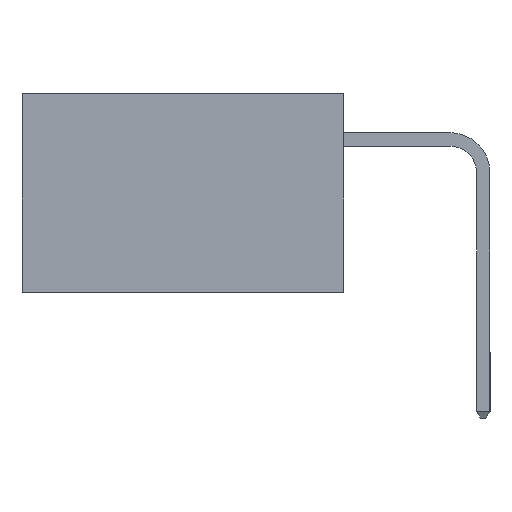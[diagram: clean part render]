
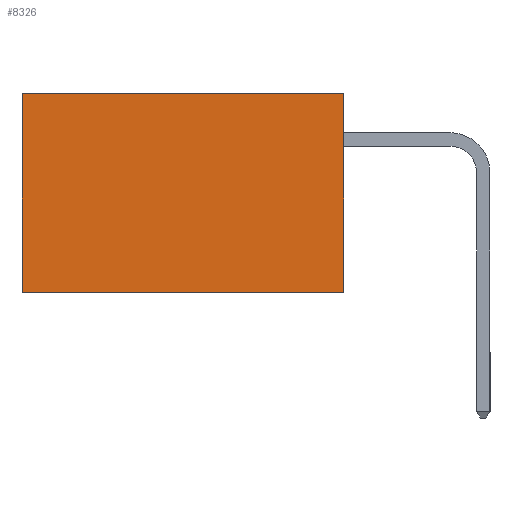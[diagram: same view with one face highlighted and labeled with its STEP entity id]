
A CAD part, left-side view. The second image highlights one B-rep face of the part: STEP entity #8326.
In plain terms, the highlighted planar face has unit normal (-1, 0, 0).
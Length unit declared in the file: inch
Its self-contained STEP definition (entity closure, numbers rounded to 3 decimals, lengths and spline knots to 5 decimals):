
#190 = ORIENTED_EDGE ( 'NONE', *, *, #11918, .T. ) ;
#529 = VECTOR ( 'NONE', #6124, 39.37008 ) ;
#577 = CARTESIAN_POINT ( 'NONE',  ( 0.2615, 0., -0.37 ) ) ;
#849 = LINE ( 'NONE', #4557, #6924 ) ;
#1777 = VERTEX_POINT ( 'NONE', #5618 ) ;
#2087 = DIRECTION ( 'NONE',  ( 0., 1., 0. ) ) ;
#2812 = VECTOR ( 'NONE', #5558, 39.37008 ) ;
#2943 = ORIENTED_EDGE ( 'NONE', *, *, #10441, .T. ) ;
#3021 = CARTESIAN_POINT ( 'NONE',  ( 0.2615, 0., -0.37 ) ) ;
#3603 = EDGE_CURVE ( 'NONE', #6421, #6858, #5610, .T. ) ;
#4172 = CARTESIAN_POINT ( 'NONE',  ( 0.2615, 0.6, -0.37 ) ) ;
#4557 = CARTESIAN_POINT ( 'NONE',  ( 0.2615, 0.6, -0.37 ) ) ;
#5007 = DIRECTION ( 'NONE',  ( 0., 0., -1. ) ) ;
#5544 = CARTESIAN_POINT ( 'NONE',  ( 0.2615, 0., -0.37 ) ) ;
#5558 = DIRECTION ( 'NONE',  ( 0., 0., -1. ) ) ;
#5610 = LINE ( 'NONE', #5544, #5855 ) ;
#5618 = CARTESIAN_POINT ( 'NONE',  ( 0.2615, 0.6, 0. ) ) ;
#5855 = VECTOR ( 'NONE', #2087, 39.37008 ) ;
#5917 = FACE_OUTER_BOUND ( 'NONE', #8085, .T. ) ;
#6124 = DIRECTION ( 'NONE',  ( 0., 1., 0. ) ) ;
#6421 = VERTEX_POINT ( 'NONE', #8128 ) ;
#6769 = ORIENTED_EDGE ( 'NONE', *, *, #8124, .F. ) ;
#6772 = PLANE ( 'NONE',  #7582 ) ;
#6858 = VERTEX_POINT ( 'NONE', #4172 ) ;
#6924 = VECTOR ( 'NONE', #8260, 39.37008 ) ;
#7440 = ORIENTED_EDGE ( 'NONE', *, *, #3603, .F. ) ;
#7582 = AXIS2_PLACEMENT_3D ( 'NONE', #3021, #8595, #5007 ) ;
#7611 = CARTESIAN_POINT ( 'NONE',  ( 0.2615, 0., 0. ) ) ;
#8015 = LINE ( 'NONE', #10806, #529 ) ;
#8085 = EDGE_LOOP ( 'NONE', ( #190, #7440, #6769, #2943 ) ) ;
#8124 = EDGE_CURVE ( 'NONE', #11503, #6421, #8899, .T. ) ;
#8128 = CARTESIAN_POINT ( 'NONE',  ( 0.2615, 0., -0.37 ) ) ;
#8260 = DIRECTION ( 'NONE',  ( 0., 0., -1. ) ) ;
#8326 = ADVANCED_FACE ( 'NONE', ( #5917 ), #6772, .F. ) ;
#8595 = DIRECTION ( 'NONE',  ( 1., 0., 0. ) ) ;
#8899 = LINE ( 'NONE', #577, #2812 ) ;
#10441 = EDGE_CURVE ( 'NONE', #11503, #1777, #8015, .T. ) ;
#10806 = CARTESIAN_POINT ( 'NONE',  ( 0.2615, 0., 0. ) ) ;
#11503 = VERTEX_POINT ( 'NONE', #7611 ) ;
#11918 = EDGE_CURVE ( 'NONE', #1777, #6858, #849, .T. ) ;
